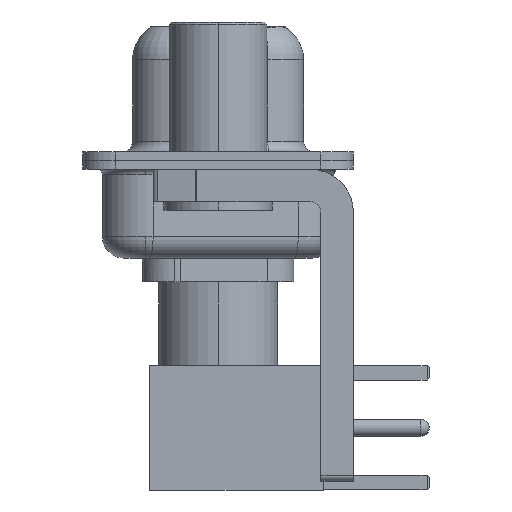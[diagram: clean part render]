
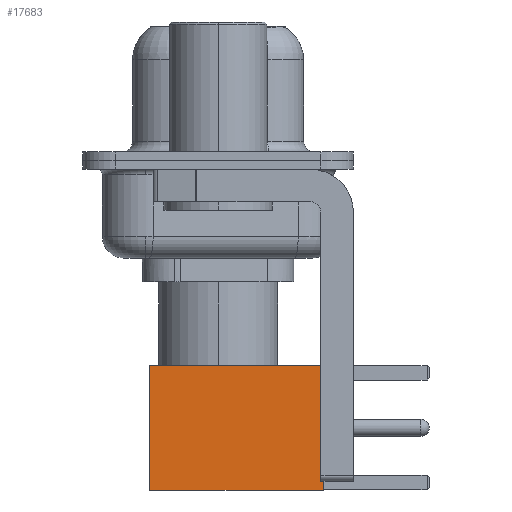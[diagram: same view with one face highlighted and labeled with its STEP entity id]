
A CAD part, left-side view. The second image highlights one B-rep face of the part: STEP entity #17683.
In plain terms, the highlighted face is planar.
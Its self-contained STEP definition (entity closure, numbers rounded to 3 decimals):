
#77 = PLANE ( 'NONE',  #2166 ) ;
#171 = CARTESIAN_POINT ( 'NONE',  ( 0., 2.875, 0. ) ) ;
#295 = VECTOR ( 'NONE', #8581, 1000. ) ;
#357 = DIRECTION ( 'NONE',  ( 0., 1., 0. ) ) ;
#989 = DIRECTION ( 'NONE',  ( -1., 0., 0. ) ) ;
#2166 = AXIS2_PLACEMENT_3D ( 'NONE', #15362, #357, #8420 ) ;
#3415 = CARTESIAN_POINT ( 'NONE',  ( -2.875, 2.875, 0. ) ) ;
#3432 = ORIENTED_EDGE ( 'NONE', *, *, #13346, .T. ) ;
#3575 = VECTOR ( 'NONE', #14843, 1000. ) ;
#4687 = CARTESIAN_POINT ( 'NONE',  ( -2.875, 2.875, 8. ) ) ;
#4956 = CARTESIAN_POINT ( 'NONE',  ( -2.875, 2.875, 0. ) ) ;
#4976 = EDGE_CURVE ( 'NONE', #9209, #12661, #12348, .T. ) ;
#5588 = FACE_OUTER_BOUND ( 'NONE', #15432, .T. ) ;
#6158 = ORIENTED_EDGE ( 'NONE', *, *, #4976, .F. ) ;
#6435 = VECTOR ( 'NONE', #989, 1000. ) ;
#6937 = LINE ( 'NONE', #11170, #295 ) ;
#8420 = DIRECTION ( 'NONE',  ( 0., 0., 1. ) ) ;
#8581 = DIRECTION ( 'NONE',  ( 0., 0., -1. ) ) ;
#8859 = VECTOR ( 'NONE', #10267, 1000. ) ;
#9209 = VERTEX_POINT ( 'NONE', #12696 ) ;
#9274 = LINE ( 'NONE', #3415, #3575 ) ;
#10267 = DIRECTION ( 'NONE',  ( -1., 0., 0. ) ) ;
#11170 = CARTESIAN_POINT ( 'NONE',  ( 2.875, 2.875, 0. ) ) ;
#11505 = VERTEX_POINT ( 'NONE', #4956 ) ;
#12348 = LINE ( 'NONE', #17817, #6435 ) ;
#12661 = VERTEX_POINT ( 'NONE', #4687 ) ;
#12696 = CARTESIAN_POINT ( 'NONE',  ( 2.875, 2.875, 8. ) ) ;
#12735 = LINE ( 'NONE', #171, #8859 ) ;
#13231 = VERTEX_POINT ( 'NONE', #14906 ) ;
#13346 = EDGE_CURVE ( 'NONE', #9209, #13231, #6937, .T. ) ;
#14765 = ORIENTED_EDGE ( 'NONE', *, *, #16182, .F. ) ;
#14843 = DIRECTION ( 'NONE',  ( 0., 0., -1. ) ) ;
#14906 = CARTESIAN_POINT ( 'NONE',  ( 2.875, 2.875, 0. ) ) ;
#15362 = CARTESIAN_POINT ( 'NONE',  ( 2.875, 2.875, 0. ) ) ;
#15432 = EDGE_LOOP ( 'NONE', ( #3432, #16313, #14765, #6158 ) ) ;
#16182 = EDGE_CURVE ( 'NONE', #12661, #11505, #9274, .T. ) ;
#16313 = ORIENTED_EDGE ( 'NONE', *, *, #16497, .T. ) ;
#16497 = EDGE_CURVE ( 'NONE', #13231, #11505, #12735, .T. ) ;
#17683 = ADVANCED_FACE ( 'NONE', ( #5588 ), #77, .T. ) ;
#17817 = CARTESIAN_POINT ( 'NONE',  ( 0., 2.875, 8. ) ) ;
